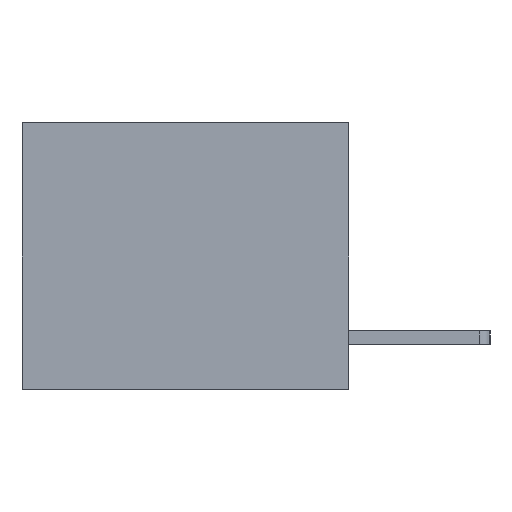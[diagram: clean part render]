
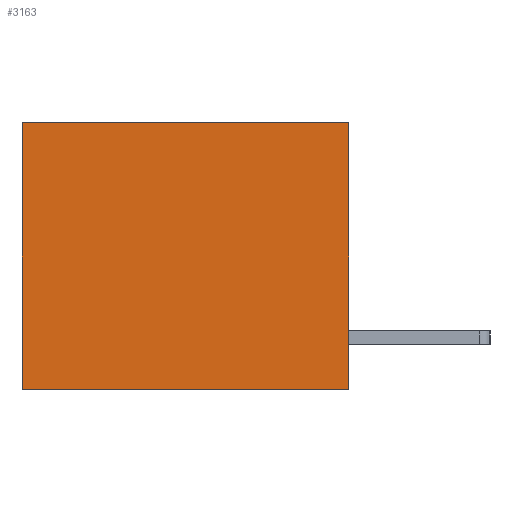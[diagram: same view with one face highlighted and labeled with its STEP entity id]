
A CAD part, left-side view. The second image highlights one B-rep face of the part: STEP entity #3163.
In plain terms, the highlighted planar face has unit normal (-1, 0, 0).
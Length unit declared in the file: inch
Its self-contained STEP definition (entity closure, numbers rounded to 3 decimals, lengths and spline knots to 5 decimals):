
#42 = DIRECTION ( 'NONE',  ( 0., 1., 0. ) ) ;
#444 = VECTOR ( 'NONE', #7860, 39.37008 ) ;
#748 = VERTEX_POINT ( 'NONE', #10754 ) ;
#1845 = FACE_OUTER_BOUND ( 'NONE', #3114, .T. ) ;
#1897 = CARTESIAN_POINT ( 'NONE',  ( 0.3165, 0., -0.49 ) ) ;
#2486 = LINE ( 'NONE', #11677, #12452 ) ;
#2676 = EDGE_CURVE ( 'NONE', #3227, #748, #10527, .T. ) ;
#3114 = EDGE_LOOP ( 'NONE', ( #5588, #10536, #4533, #4327 ) ) ;
#3163 = ADVANCED_FACE ( 'NONE', ( #1845 ), #8774, .F. ) ;
#3227 = VERTEX_POINT ( 'NONE', #9137 ) ;
#3837 = CARTESIAN_POINT ( 'NONE',  ( 0.3165, 0.6, -0.49 ) ) ;
#4327 = ORIENTED_EDGE ( 'NONE', *, *, #2676, .T. ) ;
#4533 = ORIENTED_EDGE ( 'NONE', *, *, #8767, .F. ) ;
#4771 = DIRECTION ( 'NONE',  ( 1., 0., 0. ) ) ;
#5001 = VERTEX_POINT ( 'NONE', #3837 ) ;
#5347 = LINE ( 'NONE', #7086, #5826 ) ;
#5571 = DIRECTION ( 'NONE',  ( 0., 0., -1. ) ) ;
#5588 = ORIENTED_EDGE ( 'NONE', *, *, #9797, .T. ) ;
#5684 = VERTEX_POINT ( 'NONE', #1897 ) ;
#5826 = VECTOR ( 'NONE', #6046, 39.37008 ) ;
#6046 = DIRECTION ( 'NONE',  ( 0., 0., -1. ) ) ;
#6782 = CARTESIAN_POINT ( 'NONE',  ( 0.3165, 0., -0.49 ) ) ;
#7086 = CARTESIAN_POINT ( 'NONE',  ( 0.3165, 0., -0.49 ) ) ;
#7203 = CARTESIAN_POINT ( 'NONE',  ( 0.3165, 0., 0. ) ) ;
#7860 = DIRECTION ( 'NONE',  ( 0., 1., 0. ) ) ;
#8767 = EDGE_CURVE ( 'NONE', #3227, #5684, #5347, .T. ) ;
#8774 = PLANE ( 'NONE',  #10956 ) ;
#9137 = CARTESIAN_POINT ( 'NONE',  ( 0.3165, 0., 0. ) ) ;
#9233 = VECTOR ( 'NONE', #42, 39.37008 ) ;
#9310 = EDGE_CURVE ( 'NONE', #5684, #5001, #10383, .T. ) ;
#9776 = CARTESIAN_POINT ( 'NONE',  ( 0.3165, 0., -0.49 ) ) ;
#9797 = EDGE_CURVE ( 'NONE', #748, #5001, #2486, .T. ) ;
#10383 = LINE ( 'NONE', #9776, #444 ) ;
#10527 = LINE ( 'NONE', #7203, #9233 ) ;
#10536 = ORIENTED_EDGE ( 'NONE', *, *, #9310, .F. ) ;
#10754 = CARTESIAN_POINT ( 'NONE',  ( 0.3165, 0.6, 0. ) ) ;
#10843 = DIRECTION ( 'NONE',  ( 0., 0., -1. ) ) ;
#10956 = AXIS2_PLACEMENT_3D ( 'NONE', #6782, #4771, #10843 ) ;
#11677 = CARTESIAN_POINT ( 'NONE',  ( 0.3165, 0.6, -0.49 ) ) ;
#12452 = VECTOR ( 'NONE', #5571, 39.37008 ) ;
